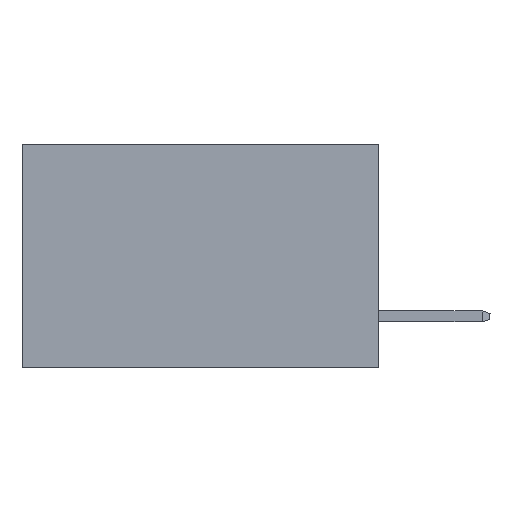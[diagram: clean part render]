
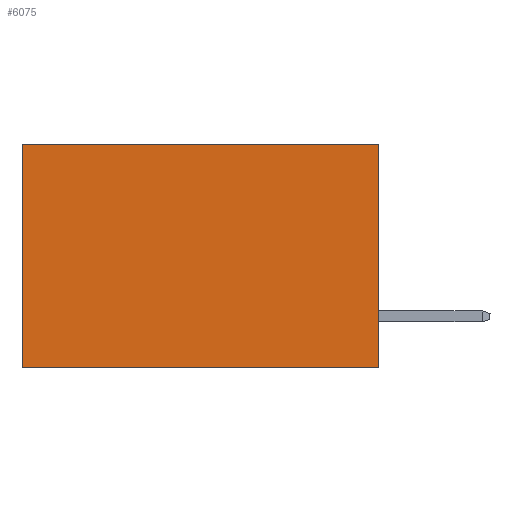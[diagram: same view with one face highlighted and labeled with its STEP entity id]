
A CAD part, left-side view. The second image highlights one B-rep face of the part: STEP entity #6075.
In plain terms, the highlighted planar face has unit normal (-1, 0, 0).
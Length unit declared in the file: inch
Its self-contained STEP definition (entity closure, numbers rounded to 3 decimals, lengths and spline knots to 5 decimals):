
#140 = EDGE_CURVE ( 'NONE', #8225, #5075, #7329, .T. ) ;
#706 = LINE ( 'NONE', #3078, #7242 ) ;
#1284 = CARTESIAN_POINT ( 'NONE',  ( 0.277, 0., -0.37 ) ) ;
#1473 = EDGE_CURVE ( 'NONE', #5075, #2530, #6605, .T. ) ;
#1811 = CARTESIAN_POINT ( 'NONE',  ( 0.277, 0., -0.37 ) ) ;
#2305 = ORIENTED_EDGE ( 'NONE', *, *, #1473, .F. ) ;
#2510 = VECTOR ( 'NONE', #2743, 39.37008 ) ;
#2530 = VERTEX_POINT ( 'NONE', #10580 ) ;
#2571 = AXIS2_PLACEMENT_3D ( 'NONE', #6197, #6172, #6155 ) ;
#2607 = ORIENTED_EDGE ( 'NONE', *, *, #8454, .T. ) ;
#2743 = DIRECTION ( 'NONE',  ( 0., 0., -1. ) ) ;
#3058 = DIRECTION ( 'NONE',  ( 0., 1., 0. ) ) ;
#3078 = CARTESIAN_POINT ( 'NONE',  ( 0.277, 0., 0. ) ) ;
#3236 = FACE_OUTER_BOUND ( 'NONE', #7896, .T. ) ;
#3958 = VECTOR ( 'NONE', #5802, 39.37008 ) ;
#4213 = PLANE ( 'NONE',  #2571 ) ;
#4552 = VECTOR ( 'NONE', #8382, 39.37008 ) ;
#4647 = CARTESIAN_POINT ( 'NONE',  ( 0.277, 0., 0. ) ) ;
#5075 = VERTEX_POINT ( 'NONE', #1811 ) ;
#5722 = CARTESIAN_POINT ( 'NONE',  ( 0.277, 0.59, -0.37 ) ) ;
#5802 = DIRECTION ( 'NONE',  ( 0., 1., 0. ) ) ;
#6075 = ADVANCED_FACE ( 'NONE', ( #3236 ), #4213, .F. ) ;
#6155 = DIRECTION ( 'NONE',  ( 0., 0., -1. ) ) ;
#6172 = DIRECTION ( 'NONE',  ( 1., 0., 0. ) ) ;
#6197 = CARTESIAN_POINT ( 'NONE',  ( 0.277, 0., -0.37 ) ) ;
#6605 = LINE ( 'NONE', #10900, #3958 ) ;
#6904 = LINE ( 'NONE', #5722, #4552 ) ;
#7242 = VECTOR ( 'NONE', #3058, 39.37008 ) ;
#7329 = LINE ( 'NONE', #1284, #2510 ) ;
#7896 = EDGE_LOOP ( 'NONE', ( #11468, #2305, #9488, #2607 ) ) ;
#8225 = VERTEX_POINT ( 'NONE', #4647 ) ;
#8382 = DIRECTION ( 'NONE',  ( 0., 0., -1. ) ) ;
#8454 = EDGE_CURVE ( 'NONE', #8225, #11257, #706, .T. ) ;
#9228 = CARTESIAN_POINT ( 'NONE',  ( 0.277, 0.59, 0. ) ) ;
#9488 = ORIENTED_EDGE ( 'NONE', *, *, #140, .F. ) ;
#10547 = EDGE_CURVE ( 'NONE', #11257, #2530, #6904, .T. ) ;
#10580 = CARTESIAN_POINT ( 'NONE',  ( 0.277, 0.59, -0.37 ) ) ;
#10900 = CARTESIAN_POINT ( 'NONE',  ( 0.277, 0., -0.37 ) ) ;
#11257 = VERTEX_POINT ( 'NONE', #9228 ) ;
#11468 = ORIENTED_EDGE ( 'NONE', *, *, #10547, .T. ) ;
